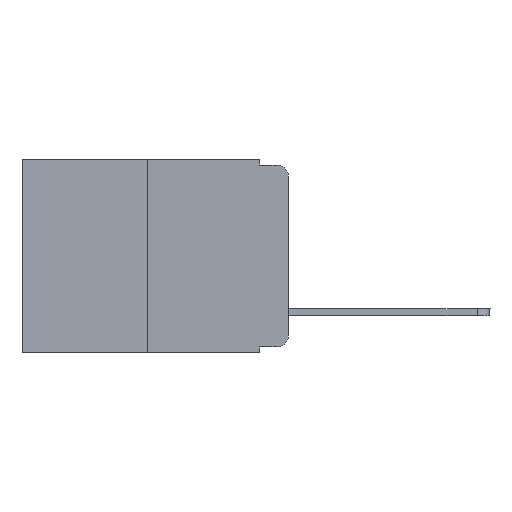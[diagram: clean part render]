
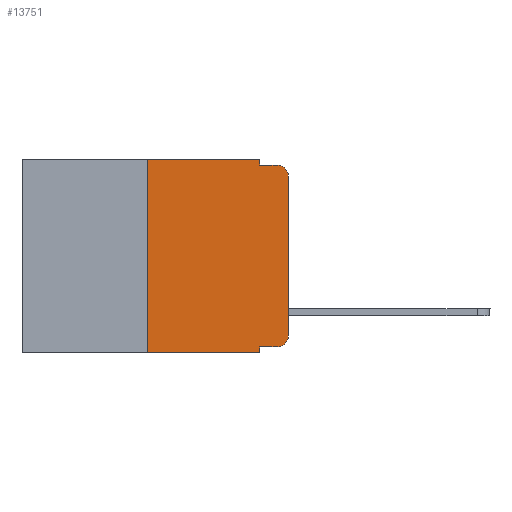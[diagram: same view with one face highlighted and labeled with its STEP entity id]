
A CAD part, left-side view. The second image highlights one B-rep face of the part: STEP entity #13751.
In plain terms, the highlighted planar face has unit normal (-1, 0, 0).
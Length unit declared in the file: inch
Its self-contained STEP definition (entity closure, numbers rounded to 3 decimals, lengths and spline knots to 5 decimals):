
#251 = ORIENTED_EDGE ( 'NONE', *, *, #2029, .F. ) ;
#289 = DIRECTION ( 'NONE',  ( 0., 0., -1. ) ) ;
#448 = CARTESIAN_POINT ( 'NONE',  ( 0., 0.02, -0.03 ) ) ;
#1026 = CARTESIAN_POINT ( 'NONE',  ( 0., 0.25, 0. ) ) ;
#1211 = LINE ( 'NONE', #9325, #3694 ) ;
#1400 = LINE ( 'NONE', #9595, #8491 ) ;
#1496 = ORIENTED_EDGE ( 'NONE', *, *, #9861, .T. ) ;
#1569 = VECTOR ( 'NONE', #6441, 39.37008 ) ;
#1792 = CARTESIAN_POINT ( 'NONE',  ( 0., 0.473, 0. ) ) ;
#1944 = DIRECTION ( 'NONE',  ( 0., 0., -1. ) ) ;
#2029 = EDGE_CURVE ( 'NONE', #14663, #9031, #3670, .T. ) ;
#2046 = LINE ( 'NONE', #7486, #9876 ) ;
#2091 = AXIS2_PLACEMENT_3D ( 'NONE', #1792, #9991, #289 ) ;
#2260 = AXIS2_PLACEMENT_3D ( 'NONE', #448, #12803, #4248 ) ;
#2389 = EDGE_CURVE ( 'NONE', #14386, #4587, #11696, .T. ) ;
#2590 = DIRECTION ( 'NONE',  ( 0., -1., 0. ) ) ;
#2818 = ORIENTED_EDGE ( 'NONE', *, *, #7893, .T. ) ;
#3522 = CARTESIAN_POINT ( 'NONE',  ( 0., 0.051, -0.01 ) ) ;
#3523 = EDGE_LOOP ( 'NONE', ( #16902, #8139, #8933, #14455, #14105, #251, #14474, #14054, #1496, #2818 ) ) ;
#3670 = LINE ( 'NONE', #1026, #1569 ) ;
#3694 = VECTOR ( 'NONE', #10737, 39.37008 ) ;
#3959 = CARTESIAN_POINT ( 'NONE',  ( 0., 0.051, 0. ) ) ;
#4159 = EDGE_CURVE ( 'NONE', #14663, #11733, #2046, .T. ) ;
#4248 = DIRECTION ( 'NONE',  ( 0., 0., -1. ) ) ;
#4307 = CIRCLE ( 'NONE', #12832, 0.02 ) ;
#4587 = VERTEX_POINT ( 'NONE', #6857 ) ;
#5068 = CARTESIAN_POINT ( 'NONE',  ( 0., 0.051, -0.333 ) ) ;
#5679 = LINE ( 'NONE', #7936, #11391 ) ;
#5964 = VECTOR ( 'NONE', #8882, 39.37008 ) ;
#5997 = DIRECTION ( 'NONE',  ( 0., -1., 0. ) ) ;
#6196 = VERTEX_POINT ( 'NONE', #7100 ) ;
#6441 = DIRECTION ( 'NONE',  ( 0., 0., 1. ) ) ;
#6595 = EDGE_CURVE ( 'NONE', #9031, #13022, #5679, .T. ) ;
#6602 = DIRECTION ( 'NONE',  ( 0., 0., -1. ) ) ;
#6857 = CARTESIAN_POINT ( 'NONE',  ( 0., 0.02, -0.01 ) ) ;
#7021 = VERTEX_POINT ( 'NONE', #7086 ) ;
#7086 = CARTESIAN_POINT ( 'NONE',  ( 0., 0., -0.03 ) ) ;
#7100 = CARTESIAN_POINT ( 'NONE',  ( 0., 0.02, -0.333 ) ) ;
#7486 = CARTESIAN_POINT ( 'NONE',  ( 0., 0.473, -0.343 ) ) ;
#7893 = EDGE_CURVE ( 'NONE', #6196, #15887, #4307, .T. ) ;
#7936 = CARTESIAN_POINT ( 'NONE',  ( 0., 0.473, 0. ) ) ;
#8139 = ORIENTED_EDGE ( 'NONE', *, *, #9756, .T. ) ;
#8491 = VECTOR ( 'NONE', #11010, 39.37008 ) ;
#8664 = VECTOR ( 'NONE', #5997, 39.37008 ) ;
#8680 = CARTESIAN_POINT ( 'NONE',  ( 0., 0.051, -0.343 ) ) ;
#8701 = CARTESIAN_POINT ( 'NONE',  ( 0., 0.051, 0. ) ) ;
#8882 = DIRECTION ( 'NONE',  ( 0., -1., 0. ) ) ;
#8933 = ORIENTED_EDGE ( 'NONE', *, *, #2389, .F. ) ;
#9031 = VERTEX_POINT ( 'NONE', #11953 ) ;
#9036 = VERTEX_POINT ( 'NONE', #11772 ) ;
#9325 = CARTESIAN_POINT ( 'NONE',  ( 0., 0.051, 0. ) ) ;
#9387 = CIRCLE ( 'NONE', #2260, 0.02 ) ;
#9595 = CARTESIAN_POINT ( 'NONE',  ( 0., 0., 0. ) ) ;
#9756 = EDGE_CURVE ( 'NONE', #7021, #4587, #9387, .T. ) ;
#9861 = EDGE_CURVE ( 'NONE', #9036, #6196, #14495, .T. ) ;
#9876 = VECTOR ( 'NONE', #11591, 39.37008 ) ;
#9904 = PLANE ( 'NONE',  #2091 ) ;
#9991 = DIRECTION ( 'NONE',  ( 1., 0., 0. ) ) ;
#10737 = DIRECTION ( 'NONE',  ( 0., 0., -1. ) ) ;
#10866 = CARTESIAN_POINT ( 'NONE',  ( 0., 0.02, -0.313 ) ) ;
#11010 = DIRECTION ( 'NONE',  ( 0., 0., 1. ) ) ;
#11389 = EDGE_CURVE ( 'NONE', #13022, #14386, #15482, .T. ) ;
#11391 = VECTOR ( 'NONE', #2590, 39.37008 ) ;
#11591 = DIRECTION ( 'NONE',  ( 0., -1., 0. ) ) ;
#11678 = EDGE_CURVE ( 'NONE', #15887, #7021, #1400, .T. ) ;
#11696 = LINE ( 'NONE', #15629, #8664 ) ;
#11733 = VERTEX_POINT ( 'NONE', #8680 ) ;
#11772 = CARTESIAN_POINT ( 'NONE',  ( 0., 0.051, -0.333 ) ) ;
#11953 = CARTESIAN_POINT ( 'NONE',  ( 0., 0.25, 0. ) ) ;
#12464 = FACE_OUTER_BOUND ( 'NONE', #3523, .T. ) ;
#12803 = DIRECTION ( 'NONE',  ( -1., 0., 0. ) ) ;
#12832 = AXIS2_PLACEMENT_3D ( 'NONE', #10866, #16244, #6602 ) ;
#13022 = VERTEX_POINT ( 'NONE', #3959 ) ;
#13094 = EDGE_CURVE ( 'NONE', #9036, #11733, #1211, .T. ) ;
#13521 = CARTESIAN_POINT ( 'NONE',  ( 0., 0.25, -0.343 ) ) ;
#13705 = CARTESIAN_POINT ( 'NONE',  ( 0., 0., -0.313 ) ) ;
#13751 = ADVANCED_FACE ( 'NONE', ( #12464 ), #9904, .F. ) ;
#14054 = ORIENTED_EDGE ( 'NONE', *, *, #13094, .F. ) ;
#14105 = ORIENTED_EDGE ( 'NONE', *, *, #6595, .F. ) ;
#14386 = VERTEX_POINT ( 'NONE', #3522 ) ;
#14455 = ORIENTED_EDGE ( 'NONE', *, *, #11389, .F. ) ;
#14474 = ORIENTED_EDGE ( 'NONE', *, *, #4159, .T. ) ;
#14495 = LINE ( 'NONE', #5068, #5964 ) ;
#14663 = VERTEX_POINT ( 'NONE', #13521 ) ;
#15482 = LINE ( 'NONE', #8701, #16328 ) ;
#15629 = CARTESIAN_POINT ( 'NONE',  ( 0., 0.051, -0.01 ) ) ;
#15887 = VERTEX_POINT ( 'NONE', #13705 ) ;
#16244 = DIRECTION ( 'NONE',  ( -1., 0., 0. ) ) ;
#16328 = VECTOR ( 'NONE', #1944, 39.37008 ) ;
#16902 = ORIENTED_EDGE ( 'NONE', *, *, #11678, .T. ) ;
